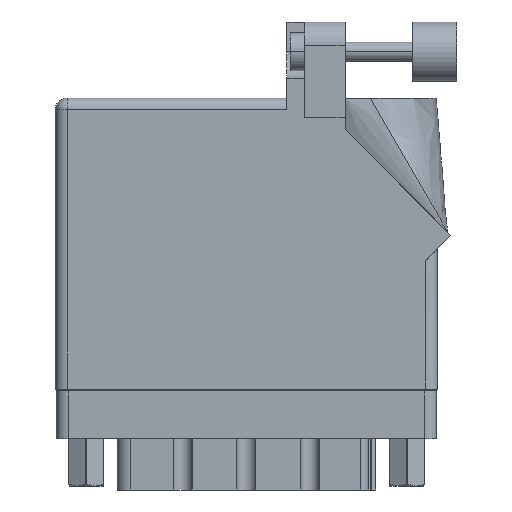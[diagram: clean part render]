
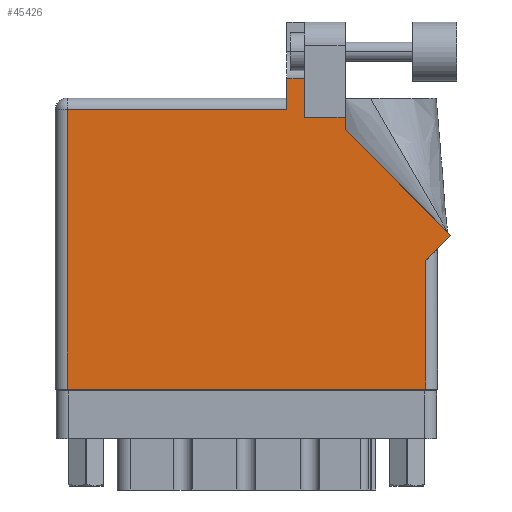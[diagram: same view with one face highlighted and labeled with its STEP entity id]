
A CAD part, front view. The second image highlights one B-rep face of the part: STEP entity #45426.
In plain terms, the highlighted face is planar.
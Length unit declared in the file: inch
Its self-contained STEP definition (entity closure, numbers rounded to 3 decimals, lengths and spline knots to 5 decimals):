
#176 = EDGE_LOOP ( 'NONE', ( #4252, #9259, #34736, #15369, #29538, #3558, #45295, #30697, #4963, #49750, #38875 ) ) ;
#1066 = CARTESIAN_POINT ( 'NONE',  ( 0.062, 0., 0. ) ) ;
#1515 = CARTESIAN_POINT ( 'NONE',  ( 1.524, 1.36442, 0. ) ) ;
#2462 = VERTEX_POINT ( 'NONE', #1515 ) ;
#3238 = VERTEX_POINT ( 'NONE', #37351 ) ;
#3259 = DIRECTION ( 'NONE',  ( -1., 0., 0. ) ) ;
#3539 = EDGE_CURVE ( 'NONE', #4355, #46456, #34826, .T. ) ;
#3558 = ORIENTED_EDGE ( 'NONE', *, *, #45057, .T. ) ;
#3635 = LINE ( 'NONE', #19180, #32704 ) ;
#4252 = ORIENTED_EDGE ( 'NONE', *, *, #29267, .T. ) ;
#4355 = VERTEX_POINT ( 'NONE', #35239 ) ;
#4773 = CARTESIAN_POINT ( 'NONE',  ( 1.217, 1.53, 0. ) ) ;
#4951 = CARTESIAN_POINT ( 'NONE',  ( 2.08071, 0.80771, 0. ) ) ;
#4963 = ORIENTED_EDGE ( 'NONE', *, *, #49872, .T. ) ;
#5198 = VERTEX_POINT ( 'NONE', #32912 ) ;
#5832 = DIRECTION ( 'NONE',  ( 0., 1., 0. ) ) ;
#7488 = DIRECTION ( 'NONE',  ( 0., 1., 0. ) ) ;
#8123 = VECTOR ( 'NONE', #8653, 39.37008 ) ;
#8254 = DIRECTION ( 'NONE',  ( 0., -1., 0. ) ) ;
#8653 = DIRECTION ( 'NONE',  ( 0., -1., 0. ) ) ;
#8862 = LINE ( 'NONE', #39051, #50117 ) ;
#9259 = ORIENTED_EDGE ( 'NONE', *, *, #39053, .T. ) ;
#10585 = CARTESIAN_POINT ( 'NONE',  ( 2.01, 0.737, 0. ) ) ;
#10756 = PLANE ( 'NONE',  #49383 ) ;
#10866 = CARTESIAN_POINT ( 'NONE',  ( 0., 1.468, 0. ) ) ;
#10911 = VERTEX_POINT ( 'NONE', #19996 ) ;
#11612 = DIRECTION ( 'NONE',  ( -1., 0., 0. ) ) ;
#13702 = VECTOR ( 'NONE', #31095, 39.37008 ) ;
#15369 = ORIENTED_EDGE ( 'NONE', *, *, #31767, .T. ) ;
#16627 = CARTESIAN_POINT ( 'NONE',  ( 1.217, 1.468, 0. ) ) ;
#18739 = CARTESIAN_POINT ( 'NONE',  ( 1.524, 1.43, 0. ) ) ;
#19180 = CARTESIAN_POINT ( 'NONE',  ( 1.948, 0.737, 0. ) ) ;
#19450 = LINE ( 'NONE', #18739, #47303 ) ;
#19593 = DIRECTION ( 'NONE',  ( 0.707, 0.707, 0. ) ) ;
#19996 = CARTESIAN_POINT ( 'NONE',  ( 1.948, 0.675, 0. ) ) ;
#20001 = VECTOR ( 'NONE', #5832, 39.37008 ) ;
#20376 = LINE ( 'NONE', #46863, #13702 ) ;
#20908 = VERTEX_POINT ( 'NONE', #33998 ) ;
#21007 = LINE ( 'NONE', #25261, #45278 ) ;
#21236 = VERTEX_POINT ( 'NONE', #1066 ) ;
#22795 = FACE_OUTER_BOUND ( 'NONE', #176, .T. ) ;
#25261 = CARTESIAN_POINT ( 'NONE',  ( 1.524, 1.36442, 0. ) ) ;
#26748 = EDGE_CURVE ( 'NONE', #10911, #41347, #30547, .T. ) ;
#29267 = EDGE_CURVE ( 'NONE', #46602, #5198, #40634, .T. ) ;
#29538 = ORIENTED_EDGE ( 'NONE', *, *, #39660, .T. ) ;
#30257 = DIRECTION ( 'NONE',  ( -1., 0., 0. ) ) ;
#30547 = LINE ( 'NONE', #10585, #48758 ) ;
#30697 = ORIENTED_EDGE ( 'NONE', *, *, #26748, .T. ) ;
#31095 = DIRECTION ( 'NONE',  ( 1., 0., 0. ) ) ;
#31211 = LINE ( 'NONE', #43559, #40334 ) ;
#31759 = LINE ( 'NONE', #38955, #49373 ) ;
#31767 = EDGE_CURVE ( 'NONE', #46456, #20908, #34406, .T. ) ;
#32704 = VECTOR ( 'NONE', #7488, 39.37008 ) ;
#32912 = CARTESIAN_POINT ( 'NONE',  ( 1.311, 1.6315, 0. ) ) ;
#33998 = CARTESIAN_POINT ( 'NONE',  ( 0.062, 1.468, 0. ) ) ;
#34163 = DIRECTION ( 'NONE',  ( 0., 0., -1. ) ) ;
#34406 = LINE ( 'NONE', #10866, #48372 ) ;
#34597 = EDGE_CURVE ( 'NONE', #46700, #46602, #19450, .T. ) ;
#34736 = ORIENTED_EDGE ( 'NONE', *, *, #3539, .T. ) ;
#34826 = LINE ( 'NONE', #4773, #8123 ) ;
#35011 = EDGE_CURVE ( 'NONE', #3238, #10911, #3635, .T. ) ;
#35239 = CARTESIAN_POINT ( 'NONE',  ( 1.217, 1.6315, 0. ) ) ;
#37351 = CARTESIAN_POINT ( 'NONE',  ( 1.948, 0., 0. ) ) ;
#37624 = CARTESIAN_POINT ( 'NONE',  ( 1.524, 1.43, 0. ) ) ;
#38875 = ORIENTED_EDGE ( 'NONE', *, *, #34597, .T. ) ;
#38955 = CARTESIAN_POINT ( 'NONE',  ( 0.062, 0., 0. ) ) ;
#39051 = CARTESIAN_POINT ( 'NONE',  ( 2.08071, 0.80771, 0. ) ) ;
#39053 = EDGE_CURVE ( 'NONE', #5198, #4355, #31211, .T. ) ;
#39660 = EDGE_CURVE ( 'NONE', #20908, #21236, #31759, .T. ) ;
#40334 = VECTOR ( 'NONE', #43403, 39.37008 ) ;
#40634 = LINE ( 'NONE', #44469, #20001 ) ;
#41347 = VERTEX_POINT ( 'NONE', #4951 ) ;
#43403 = DIRECTION ( 'NONE',  ( -1., 0., 0. ) ) ;
#43441 = DIRECTION ( 'NONE',  ( -0.707, 0.707, 0. ) ) ;
#43559 = CARTESIAN_POINT ( 'NONE',  ( 1.64177, 1.6315, 0. ) ) ;
#44469 = CARTESIAN_POINT ( 'NONE',  ( 1.311, 1.43, 0. ) ) ;
#44712 = EDGE_CURVE ( 'NONE', #2462, #46700, #21007, .T. ) ;
#44909 = CARTESIAN_POINT ( 'NONE',  ( 1.311, 1.43, 0. ) ) ;
#45057 = EDGE_CURVE ( 'NONE', #21236, #3238, #20376, .T. ) ;
#45278 = VECTOR ( 'NONE', #48258, 39.37008 ) ;
#45295 = ORIENTED_EDGE ( 'NONE', *, *, #35011, .T. ) ;
#45426 = ADVANCED_FACE ( 'NONE', ( #22795 ), #10756, .F. ) ;
#46211 = CARTESIAN_POINT ( 'NONE',  ( 0., 1.53, 0. ) ) ;
#46456 = VERTEX_POINT ( 'NONE', #16627 ) ;
#46602 = VERTEX_POINT ( 'NONE', #44909 ) ;
#46700 = VERTEX_POINT ( 'NONE', #37624 ) ;
#46863 = CARTESIAN_POINT ( 'NONE',  ( 0., 0., 0. ) ) ;
#47303 = VECTOR ( 'NONE', #11612, 39.37008 ) ;
#48258 = DIRECTION ( 'NONE',  ( 0., 1., 0. ) ) ;
#48372 = VECTOR ( 'NONE', #3259, 39.37008 ) ;
#48758 = VECTOR ( 'NONE', #19593, 39.37008 ) ;
#49373 = VECTOR ( 'NONE', #8254, 39.37008 ) ;
#49383 = AXIS2_PLACEMENT_3D ( 'NONE', #46211, #34163, #30257 ) ;
#49750 = ORIENTED_EDGE ( 'NONE', *, *, #44712, .T. ) ;
#49872 = EDGE_CURVE ( 'NONE', #41347, #2462, #8862, .T. ) ;
#50117 = VECTOR ( 'NONE', #43441, 39.37008 ) ;
